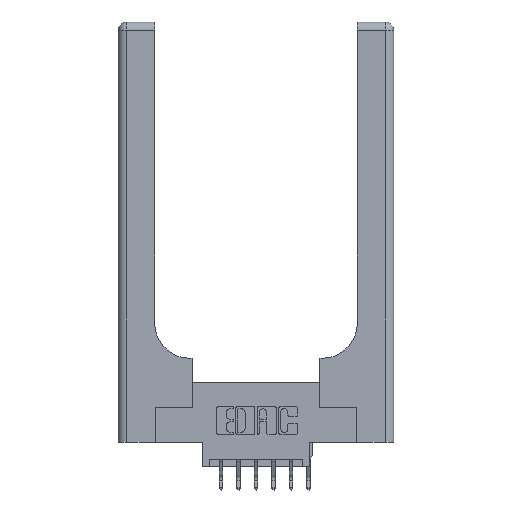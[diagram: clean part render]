
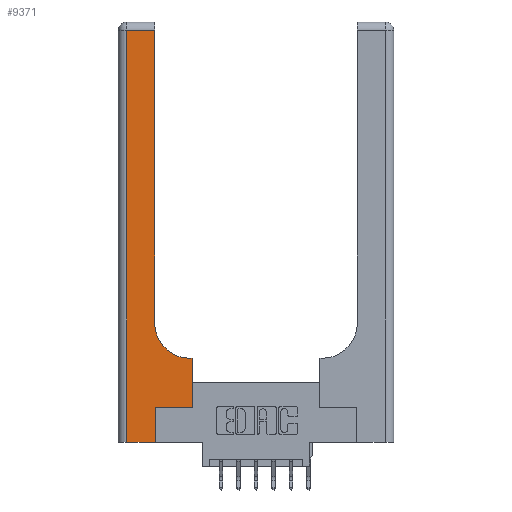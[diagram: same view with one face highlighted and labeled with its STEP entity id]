
A CAD part, top view. The second image highlights one B-rep face of the part: STEP entity #9371.
In plain terms, the highlighted planar face has unit normal (0, 0, 1).
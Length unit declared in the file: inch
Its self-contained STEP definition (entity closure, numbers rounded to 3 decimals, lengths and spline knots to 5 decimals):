
#18 = DIRECTION ( 'NONE',  ( 0., -1., 0. ) ) ;
#103 = VERTEX_POINT ( 'NONE', #4817 ) ;
#132 = EDGE_CURVE ( 'NONE', #1654, #103, #11740, .T. ) ;
#455 = CIRCLE ( 'NONE', #5285, 0.25 ) ;
#1030 = CARTESIAN_POINT ( 'NONE',  ( 0.06, 3., 0.37 ) ) ;
#1464 = VECTOR ( 'NONE', #4781, 39.37008 ) ;
#1654 = VERTEX_POINT ( 'NONE', #5686 ) ;
#1698 = ORIENTED_EDGE ( 'NONE', *, *, #132, .T. ) ;
#1834 = LINE ( 'NONE', #10662, #6790 ) ;
#1847 = FACE_OUTER_BOUND ( 'NONE', #12263, .T. ) ;
#1903 = ORIENTED_EDGE ( 'NONE', *, *, #12671, .T. ) ;
#2385 = CARTESIAN_POINT ( 'NONE',  ( 0.26, 2.94, 0.37 ) ) ;
#2706 = VECTOR ( 'NONE', #11888, 39.37008 ) ;
#2713 = ORIENTED_EDGE ( 'NONE', *, *, #4841, .T. ) ;
#3205 = ORIENTED_EDGE ( 'NONE', *, *, #3834, .T. ) ;
#3413 = ORIENTED_EDGE ( 'NONE', *, *, #9558, .T. ) ;
#3834 = EDGE_CURVE ( 'NONE', #103, #8463, #12305, .T. ) ;
#3861 = ORIENTED_EDGE ( 'NONE', *, *, #7630, .T. ) ;
#3981 = VERTEX_POINT ( 'NONE', #12676 ) ;
#4065 = CARTESIAN_POINT ( 'NONE',  ( 0., 3., 0.37 ) ) ;
#4458 = VERTEX_POINT ( 'NONE', #8246 ) ;
#4496 = DIRECTION ( 'NONE',  ( 1., 0., 0. ) ) ;
#4675 = CARTESIAN_POINT ( 'NONE',  ( 0., 2.94, 0.37 ) ) ;
#4781 = DIRECTION ( 'NONE',  ( 1., 0., 0. ) ) ;
#4817 = CARTESIAN_POINT ( 'NONE',  ( 0.265, 0.25, 0.37 ) ) ;
#4841 = EDGE_CURVE ( 'NONE', #11875, #3981, #7989, .T. ) ;
#4921 = VECTOR ( 'NONE', #8641, 39.37008 ) ;
#5152 = CARTESIAN_POINT ( 'NONE',  ( 0.265, 0., 0.37 ) ) ;
#5220 = CARTESIAN_POINT ( 'NONE',  ( 0.528, 0.6, 0.37 ) ) ;
#5285 = AXIS2_PLACEMENT_3D ( 'NONE', #7979, #6809, #4496 ) ;
#5303 = ORIENTED_EDGE ( 'NONE', *, *, #10815, .T. ) ;
#5360 = VERTEX_POINT ( 'NONE', #2385 ) ;
#5686 = CARTESIAN_POINT ( 'NONE',  ( 0.265, 0., 0.37 ) ) ;
#5985 = DIRECTION ( 'NONE',  ( 1., 0., 0. ) ) ;
#6011 = CARTESIAN_POINT ( 'NONE',  ( 0.06, 0., 0.37 ) ) ;
#6450 = LINE ( 'NONE', #7472, #4921 ) ;
#6547 = VECTOR ( 'NONE', #10388, 39.37008 ) ;
#6790 = VECTOR ( 'NONE', #7244, 39.37008 ) ;
#6809 = DIRECTION ( 'NONE',  ( 0., 0., -1. ) ) ;
#6852 = LINE ( 'NONE', #4675, #9159 ) ;
#6922 = DIRECTION ( 'NONE',  ( -1., 0., 0. ) ) ;
#7244 = DIRECTION ( 'NONE',  ( 0., 1., 0. ) ) ;
#7367 = CARTESIAN_POINT ( 'NONE',  ( 0.528, 0.25, 0.37 ) ) ;
#7472 = CARTESIAN_POINT ( 'NONE',  ( 0.528, 0.25, 0.37 ) ) ;
#7600 = LINE ( 'NONE', #1030, #8286 ) ;
#7630 = EDGE_CURVE ( 'NONE', #5360, #12893, #6852, .T. ) ;
#7781 = DIRECTION ( 'NONE',  ( -1., 0., 0. ) ) ;
#7979 = CARTESIAN_POINT ( 'NONE',  ( 0.51, 0.85, 0.37 ) ) ;
#7989 = LINE ( 'NONE', #8133, #6547 ) ;
#8133 = CARTESIAN_POINT ( 'NONE',  ( 0.26, 0.6, 0.37 ) ) ;
#8246 = CARTESIAN_POINT ( 'NONE',  ( 0.26, 0.85, 0.37 ) ) ;
#8286 = VECTOR ( 'NONE', #18, 39.37008 ) ;
#8401 = AXIS2_PLACEMENT_3D ( 'NONE', #4065, #8501, #7781 ) ;
#8463 = VERTEX_POINT ( 'NONE', #7367 ) ;
#8501 = DIRECTION ( 'NONE',  ( 0., 0., -1. ) ) ;
#8641 = DIRECTION ( 'NONE',  ( 0., 1., 0. ) ) ;
#9159 = VECTOR ( 'NONE', #6922, 39.37008 ) ;
#9371 = ADVANCED_FACE ( 'NONE', ( #1847 ), #13996, .F. ) ;
#9558 = EDGE_CURVE ( 'NONE', #4458, #5360, #1834, .T. ) ;
#9595 = VERTEX_POINT ( 'NONE', #6011 ) ;
#9649 = ORIENTED_EDGE ( 'NONE', *, *, #10892, .T. ) ;
#10388 = DIRECTION ( 'NONE',  ( -1., 0., 0. ) ) ;
#10662 = CARTESIAN_POINT ( 'NONE',  ( 0.26, 3., 0.37 ) ) ;
#10777 = ORIENTED_EDGE ( 'NONE', *, *, #11123, .T. ) ;
#10815 = EDGE_CURVE ( 'NONE', #8463, #11875, #6450, .T. ) ;
#10892 = EDGE_CURVE ( 'NONE', #3981, #4458, #455, .T. ) ;
#11123 = EDGE_CURVE ( 'NONE', #12893, #9595, #7600, .T. ) ;
#11698 = CARTESIAN_POINT ( 'NONE',  ( 0., 0., 0.37 ) ) ;
#11740 = LINE ( 'NONE', #5152, #2706 ) ;
#11875 = VERTEX_POINT ( 'NONE', #5220 ) ;
#11888 = DIRECTION ( 'NONE',  ( 0., 1., 0. ) ) ;
#12263 = EDGE_LOOP ( 'NONE', ( #3413, #3861, #10777, #1903, #1698, #3205, #5303, #2713, #9649 ) ) ;
#12305 = LINE ( 'NONE', #13554, #1464 ) ;
#12671 = EDGE_CURVE ( 'NONE', #9595, #1654, #13668, .T. ) ;
#12676 = CARTESIAN_POINT ( 'NONE',  ( 0.51, 0.6, 0.37 ) ) ;
#12893 = VERTEX_POINT ( 'NONE', #14138 ) ;
#13554 = CARTESIAN_POINT ( 'NONE',  ( 0.265, 0.25, 0.37 ) ) ;
#13668 = LINE ( 'NONE', #11698, #14249 ) ;
#13996 = PLANE ( 'NONE',  #8401 ) ;
#14138 = CARTESIAN_POINT ( 'NONE',  ( 0.06, 2.94, 0.37 ) ) ;
#14249 = VECTOR ( 'NONE', #5985, 39.37008 ) ;
